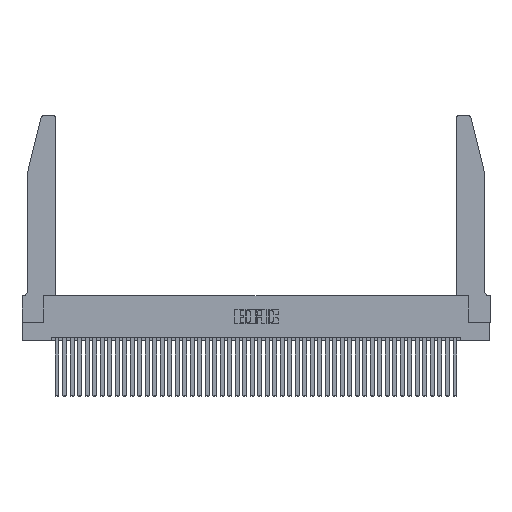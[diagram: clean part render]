
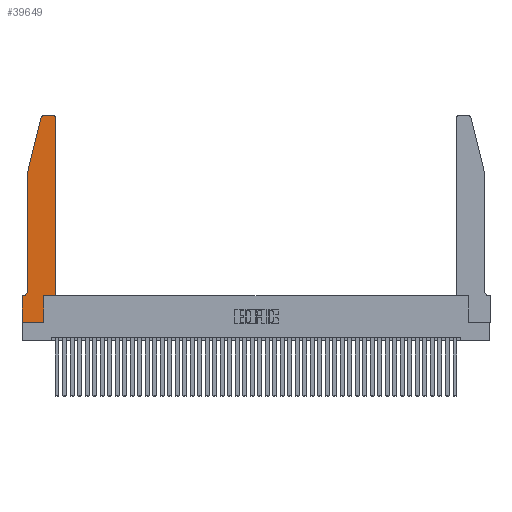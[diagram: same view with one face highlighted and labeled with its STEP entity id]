
A CAD part, top view. The second image highlights one B-rep face of the part: STEP entity #39649.
In plain terms, the highlighted planar face has unit normal (0, 0, 1).
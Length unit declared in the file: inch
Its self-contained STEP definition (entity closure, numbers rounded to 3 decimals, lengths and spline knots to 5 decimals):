
#10 = LINE ( 'NONE', #17955, #7748 ) ;
#699 = CARTESIAN_POINT ( 'NONE',  ( 0.2865, 0.35, 0.37 ) ) ;
#1179 = CARTESIAN_POINT ( 'NONE',  ( 0.25487, 2.72718, 0.37 ) ) ;
#1217 = VERTEX_POINT ( 'NONE', #13109 ) ;
#1560 = CARTESIAN_POINT ( 'NONE',  ( 0.4505, 0.35, 0.37 ) ) ;
#1761 = ORIENTED_EDGE ( 'NONE', *, *, #20644, .T. ) ;
#2193 = ORIENTED_EDGE ( 'NONE', *, *, #9993, .T. ) ;
#2266 = EDGE_CURVE ( 'NONE', #12060, #41512, #13148, .T. ) ;
#2750 = CIRCLE ( 'NONE', #44186, 0.03 ) ;
#3259 = CARTESIAN_POINT ( 'NONE',  ( 0.4505, 0.35, 0.37 ) ) ;
#3437 = EDGE_CURVE ( 'NONE', #43753, #38396, #22448, .T. ) ;
#3769 = ORIENTED_EDGE ( 'NONE', *, *, #5367, .T. ) ;
#4312 = VERTEX_POINT ( 'NONE', #28767 ) ;
#4789 = VERTEX_POINT ( 'NONE', #3259 ) ;
#4792 = EDGE_CURVE ( 'NONE', #25195, #21140, #21343, .T. ) ;
#4880 = LINE ( 'NONE', #21614, #5453 ) ;
#5367 = EDGE_CURVE ( 'NONE', #26603, #1217, #4880, .T. ) ;
#5453 = VECTOR ( 'NONE', #39498, 39.37008 ) ;
#6624 = EDGE_CURVE ( 'NONE', #4789, #34466, #20628, .T. ) ;
#7407 = CARTESIAN_POINT ( 'NONE',  ( 0., 0., 0.37 ) ) ;
#7739 = DIRECTION ( 'NONE',  ( 0., 0., -1. ) ) ;
#7748 = VECTOR ( 'NONE', #10562, 39.37008 ) ;
#8616 = DIRECTION ( 'NONE',  ( 0., 0., 1. ) ) ;
#8744 = DIRECTION ( 'NONE',  ( 1., 0., 0. ) ) ;
#8764 = CARTESIAN_POINT ( 'NONE',  ( 0.284, 2.72, 0.37 ) ) ;
#9993 = EDGE_CURVE ( 'NONE', #38396, #4789, #10, .T. ) ;
#10035 = VERTEX_POINT ( 'NONE', #21598 ) ;
#10457 = ORIENTED_EDGE ( 'NONE', *, *, #21884, .T. ) ;
#10562 = DIRECTION ( 'NONE',  ( 1., 0., 0. ) ) ;
#11006 = DIRECTION ( 'NONE',  ( 0., 1., 0. ) ) ;
#11018 = DIRECTION ( 'NONE',  ( 0., 0., 1. ) ) ;
#11896 = CARTESIAN_POINT ( 'NONE',  ( 0.0755, 0.35, 0.37 ) ) ;
#11949 = PLANE ( 'NONE',  #29439 ) ;
#11993 = EDGE_CURVE ( 'NONE', #4312, #43753, #37478, .T. ) ;
#12060 = VERTEX_POINT ( 'NONE', #1179 ) ;
#12202 = CARTESIAN_POINT ( 'NONE',  ( 0.2865, 0.35, 0.37 ) ) ;
#12771 = ORIENTED_EDGE ( 'NONE', *, *, #4792, .T. ) ;
#12842 = CARTESIAN_POINT ( 'NONE',  ( 0.0755, 0.42, 0.37 ) ) ;
#12940 = VECTOR ( 'NONE', #37109, 39.37008 ) ;
#13109 = CARTESIAN_POINT ( 'NONE',  ( 0.284, 2.75, 0.37 ) ) ;
#13148 = LINE ( 'NONE', #34141, #29550 ) ;
#14124 = VECTOR ( 'NONE', #36068, 39.37008 ) ;
#15338 = DIRECTION ( 'NONE',  ( 1., 0., 0. ) ) ;
#15471 = CARTESIAN_POINT ( 'NONE',  ( 0., 0., 0.37 ) ) ;
#15476 = CARTESIAN_POINT ( 'NONE',  ( 0., 0.35, 0.37 ) ) ;
#16017 = EDGE_LOOP ( 'NONE', ( #3769, #1761, #38353, #10457, #12771, #29452, #42597, #42242, #24650, #2193, #41243, #22943 ) ) ;
#16743 = CARTESIAN_POINT ( 'NONE',  ( 0.4205, 2.75, 0.37 ) ) ;
#16860 = EDGE_CURVE ( 'NONE', #10035, #4312, #31249, .T. ) ;
#17420 = LINE ( 'NONE', #11896, #14124 ) ;
#17514 = DIRECTION ( 'NONE',  ( 0., -1., 0. ) ) ;
#17955 = CARTESIAN_POINT ( 'NONE',  ( 0.4505, 0.35, 0.37 ) ) ;
#20628 = LINE ( 'NONE', #1560, #12940 ) ;
#20644 = EDGE_CURVE ( 'NONE', #1217, #12060, #44195, .T. ) ;
#20827 = CARTESIAN_POINT ( 'NONE',  ( 0.4505, 2.72, 0.37 ) ) ;
#21058 = DIRECTION ( 'NONE',  ( -1., 0., 0. ) ) ;
#21140 = VERTEX_POINT ( 'NONE', #42374 ) ;
#21213 = DIRECTION ( 'NONE',  ( 0., -1., 0. ) ) ;
#21343 = CIRCLE ( 'NONE', #28785, 0.07 ) ;
#21436 = CARTESIAN_POINT ( 'NONE',  ( 0.4205, 2.72, 0.37 ) ) ;
#21598 = CARTESIAN_POINT ( 'NONE',  ( 0., 0.35, 0.37 ) ) ;
#21614 = CARTESIAN_POINT ( 'NONE',  ( 0.2605, 2.75, 0.37 ) ) ;
#21884 = EDGE_CURVE ( 'NONE', #41512, #25195, #44068, .T. ) ;
#22448 = LINE ( 'NONE', #699, #26228 ) ;
#22943 = ORIENTED_EDGE ( 'NONE', *, *, #31521, .T. ) ;
#23790 = CARTESIAN_POINT ( 'NONE',  ( 0.2865, 0., 0.37 ) ) ;
#24650 = ORIENTED_EDGE ( 'NONE', *, *, #3437, .T. ) ;
#24954 = DIRECTION ( 'NONE',  ( 1., 0., 0. ) ) ;
#25195 = VERTEX_POINT ( 'NONE', #12842 ) ;
#25855 = DIRECTION ( 'NONE',  ( 0., 0., 1. ) ) ;
#26228 = VECTOR ( 'NONE', #11006, 39.37008 ) ;
#26603 = VERTEX_POINT ( 'NONE', #16743 ) ;
#27471 = CARTESIAN_POINT ( 'NONE',  ( 0.0755, 2., 0.37 ) ) ;
#28767 = CARTESIAN_POINT ( 'NONE',  ( 0., 0., 0.37 ) ) ;
#28785 = AXIS2_PLACEMENT_3D ( 'NONE', #39093, #7739, #21058 ) ;
#29207 = VECTOR ( 'NONE', #8744, 39.37008 ) ;
#29439 = AXIS2_PLACEMENT_3D ( 'NONE', #15476, #25855, #32891 ) ;
#29452 = ORIENTED_EDGE ( 'NONE', *, *, #44759, .T. ) ;
#29550 = VECTOR ( 'NONE', #33985, 39.37008 ) ;
#31249 = LINE ( 'NONE', #7407, #43843 ) ;
#31521 = EDGE_CURVE ( 'NONE', #34466, #26603, #2750, .T. ) ;
#32891 = DIRECTION ( 'NONE',  ( 1., 0., 0. ) ) ;
#33985 = DIRECTION ( 'NONE',  ( -0.239, -0.971, 0. ) ) ;
#34141 = CARTESIAN_POINT ( 'NONE',  ( 0.0755, 2., 0.37 ) ) ;
#34466 = VERTEX_POINT ( 'NONE', #20827 ) ;
#36068 = DIRECTION ( 'NONE',  ( -1., 0., 0. ) ) ;
#36965 = VECTOR ( 'NONE', #21213, 39.37008 ) ;
#37109 = DIRECTION ( 'NONE',  ( 0., 1., 0. ) ) ;
#37478 = LINE ( 'NONE', #15471, #29207 ) ;
#38353 = ORIENTED_EDGE ( 'NONE', *, *, #2266, .T. ) ;
#38396 = VERTEX_POINT ( 'NONE', #12202 ) ;
#39093 = CARTESIAN_POINT ( 'NONE',  ( 0.0055, 0.42, 0.37 ) ) ;
#39498 = DIRECTION ( 'NONE',  ( -1., 0., 0. ) ) ;
#39649 = ADVANCED_FACE ( 'NONE', ( #41889 ), #11949, .T. ) ;
#41243 = ORIENTED_EDGE ( 'NONE', *, *, #6624, .T. ) ;
#41512 = VERTEX_POINT ( 'NONE', #27471 ) ;
#41889 = FACE_OUTER_BOUND ( 'NONE', #16017, .T. ) ;
#42168 = CARTESIAN_POINT ( 'NONE',  ( 0.0755, 2., 0.37 ) ) ;
#42242 = ORIENTED_EDGE ( 'NONE', *, *, #11993, .T. ) ;
#42374 = CARTESIAN_POINT ( 'NONE',  ( 0.0055, 0.35, 0.37 ) ) ;
#42597 = ORIENTED_EDGE ( 'NONE', *, *, #16860, .T. ) ;
#42704 = AXIS2_PLACEMENT_3D ( 'NONE', #8764, #8616, #15338 ) ;
#43753 = VERTEX_POINT ( 'NONE', #23790 ) ;
#43843 = VECTOR ( 'NONE', #17514, 39.37008 ) ;
#44068 = LINE ( 'NONE', #42168, #36965 ) ;
#44186 = AXIS2_PLACEMENT_3D ( 'NONE', #21436, #11018, #24954 ) ;
#44195 = CIRCLE ( 'NONE', #42704, 0.03 ) ;
#44759 = EDGE_CURVE ( 'NONE', #21140, #10035, #17420, .T. ) ;
